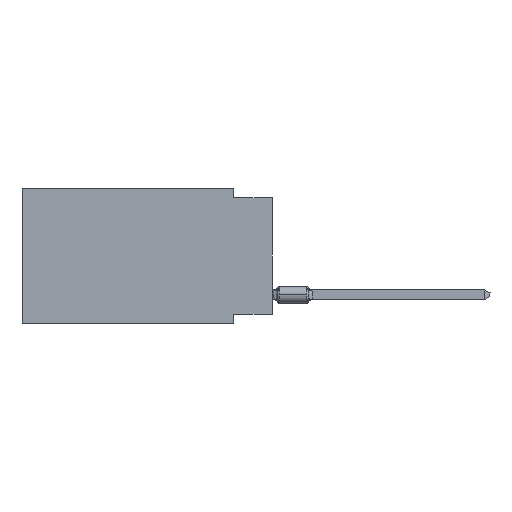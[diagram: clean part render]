
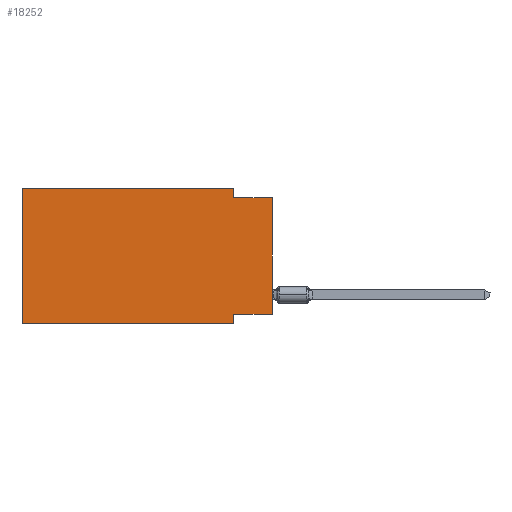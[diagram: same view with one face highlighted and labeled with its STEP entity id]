
A CAD part, left-side view. The second image highlights one B-rep face of the part: STEP entity #18252.
In plain terms, the highlighted planar face has unit normal (-1, 0, 0).
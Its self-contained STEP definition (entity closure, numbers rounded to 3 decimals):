
#1378 = CARTESIAN_POINT ( 'NONE',  ( 0., 0., -0.635 ) ) ;
#2468 = EDGE_CURVE ( 'NONE', #20157, #15937, #36761, .T. ) ;
#2515 = ORIENTED_EDGE ( 'NONE', *, *, #31073, .T. ) ;
#2712 = ORIENTED_EDGE ( 'NONE', *, *, #32992, .F. ) ;
#4300 = CARTESIAN_POINT ( 'NONE',  ( 0., 16.383, 0. ) ) ;
#5122 = EDGE_LOOP ( 'NONE', ( #22972, #33154, #16233, #22405, #6479, #2515, #29268, #2712 ) ) ;
#5270 = CARTESIAN_POINT ( 'NONE',  ( 0., 16.383, 0. ) ) ;
#6479 = ORIENTED_EDGE ( 'NONE', *, *, #18458, .F. ) ;
#7069 = CARTESIAN_POINT ( 'NONE',  ( 0., 16.383, -8.89 ) ) ;
#7215 = VECTOR ( 'NONE', #26509, 1000. ) ;
#7618 = DIRECTION ( 'NONE',  ( 0., 0., 1. ) ) ;
#8919 = CARTESIAN_POINT ( 'NONE',  ( 0., 2.54, -8.255 ) ) ;
#9995 = LINE ( 'NONE', #4300, #29521 ) ;
#10371 = DIRECTION ( 'NONE',  ( 0., -1., 0. ) ) ;
#11221 = VECTOR ( 'NONE', #27941, 1000. ) ;
#13356 = VERTEX_POINT ( 'NONE', #16276 ) ;
#13808 = CARTESIAN_POINT ( 'NONE',  ( 0., 2.54, 0. ) ) ;
#14595 = VERTEX_POINT ( 'NONE', #29363 ) ;
#15353 = DIRECTION ( 'NONE',  ( 0., 1., 0. ) ) ;
#15937 = VERTEX_POINT ( 'NONE', #34602 ) ;
#16233 = ORIENTED_EDGE ( 'NONE', *, *, #2468, .F. ) ;
#16276 = CARTESIAN_POINT ( 'NONE',  ( 0., 16.383, 0. ) ) ;
#17214 = DIRECTION ( 'NONE',  ( 1., 0., 0. ) ) ;
#18252 = ADVANCED_FACE ( 'NONE', ( #31282 ), #22718, .F. ) ;
#18458 = EDGE_CURVE ( 'NONE', #26775, #13356, #22578, .T. ) ;
#19067 = CARTESIAN_POINT ( 'NONE',  ( 0., 16.383, -8.89 ) ) ;
#20157 = VERTEX_POINT ( 'NONE', #13808 ) ;
#20737 = VERTEX_POINT ( 'NONE', #21378 ) ;
#20845 = CARTESIAN_POINT ( 'NONE',  ( 0., 0., -8.255 ) ) ;
#21089 = VECTOR ( 'NONE', #15353, 1000. ) ;
#21378 = CARTESIAN_POINT ( 'NONE',  ( 0., 2.54, -8.89 ) ) ;
#21489 = LINE ( 'NONE', #7069, #27033 ) ;
#22070 = AXIS2_PLACEMENT_3D ( 'NONE', #5270, #17214, #28813 ) ;
#22405 = ORIENTED_EDGE ( 'NONE', *, *, #24533, .F. ) ;
#22578 = LINE ( 'NONE', #25820, #34202 ) ;
#22718 = PLANE ( 'NONE',  #22070 ) ;
#22972 = ORIENTED_EDGE ( 'NONE', *, *, #32394, .T. ) ;
#24086 = LINE ( 'NONE', #20845, #21089 ) ;
#24528 = DIRECTION ( 'NONE',  ( 0., -1., 0. ) ) ;
#24533 = EDGE_CURVE ( 'NONE', #13356, #20157, #9995, .T. ) ;
#24731 = VERTEX_POINT ( 'NONE', #31603 ) ;
#24911 = LINE ( 'NONE', #33642, #32601 ) ;
#25820 = CARTESIAN_POINT ( 'NONE',  ( 0., 16.383, 0. ) ) ;
#26509 = DIRECTION ( 'NONE',  ( 0., 0., -1. ) ) ;
#26775 = VERTEX_POINT ( 'NONE', #19067 ) ;
#27033 = VECTOR ( 'NONE', #24528, 1000. ) ;
#27394 = LINE ( 'NONE', #1378, #11221 ) ;
#27517 = DIRECTION ( 'NONE',  ( 0., 0., -1. ) ) ;
#27941 = DIRECTION ( 'NONE',  ( 0., -1., 0. ) ) ;
#28491 = DIRECTION ( 'NONE',  ( 0., 0., 1. ) ) ;
#28813 = DIRECTION ( 'NONE',  ( 0., 0., -1. ) ) ;
#28820 = VECTOR ( 'NONE', #27517, 1000. ) ;
#29268 = ORIENTED_EDGE ( 'NONE', *, *, #34498, .F. ) ;
#29363 = CARTESIAN_POINT ( 'NONE',  ( 0., 0., -0.635 ) ) ;
#29521 = VECTOR ( 'NONE', #10371, 1000. ) ;
#30025 = VERTEX_POINT ( 'NONE', #8919 ) ;
#31058 = EDGE_CURVE ( 'NONE', #15937, #14595, #27394, .T. ) ;
#31073 = EDGE_CURVE ( 'NONE', #26775, #20737, #21489, .T. ) ;
#31282 = FACE_OUTER_BOUND ( 'NONE', #5122, .T. ) ;
#31603 = CARTESIAN_POINT ( 'NONE',  ( 0., 0., -8.255 ) ) ;
#32394 = EDGE_CURVE ( 'NONE', #24731, #14595, #24911, .T. ) ;
#32601 = VECTOR ( 'NONE', #7618, 1000. ) ;
#32992 = EDGE_CURVE ( 'NONE', #24731, #30025, #24086, .T. ) ;
#33154 = ORIENTED_EDGE ( 'NONE', *, *, #31058, .F. ) ;
#33642 = CARTESIAN_POINT ( 'NONE',  ( 0., 0., 0. ) ) ;
#33929 = CARTESIAN_POINT ( 'NONE',  ( 0., 2.54, -8.89 ) ) ;
#34202 = VECTOR ( 'NONE', #28491, 1000. ) ;
#34498 = EDGE_CURVE ( 'NONE', #30025, #20737, #36762, .T. ) ;
#34602 = CARTESIAN_POINT ( 'NONE',  ( 0., 2.54, -0.635 ) ) ;
#35908 = CARTESIAN_POINT ( 'NONE',  ( 0., 2.54, 0. ) ) ;
#36761 = LINE ( 'NONE', #35908, #28820 ) ;
#36762 = LINE ( 'NONE', #33929, #7215 ) ;
